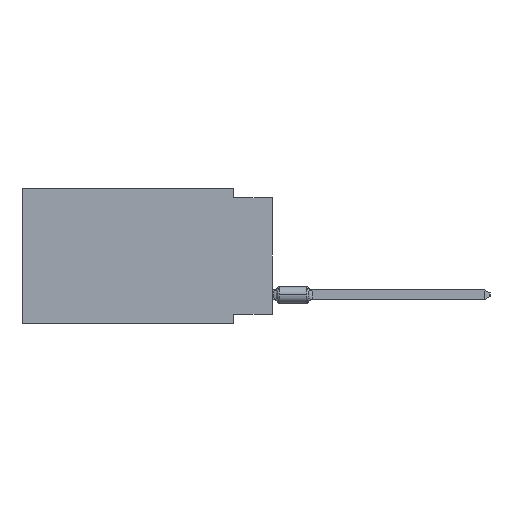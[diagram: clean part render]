
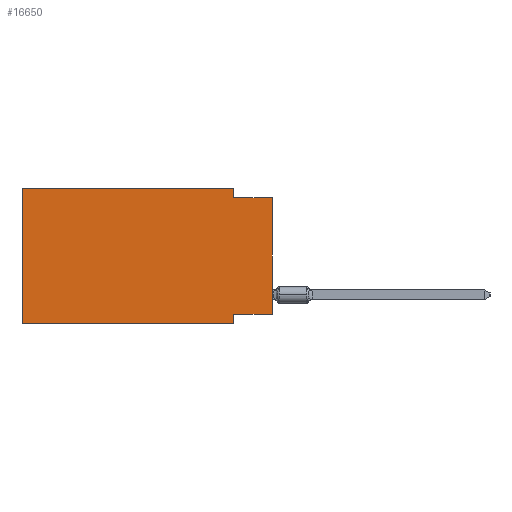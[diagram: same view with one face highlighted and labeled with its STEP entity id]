
A CAD part, left-side view. The second image highlights one B-rep face of the part: STEP entity #16650.
In plain terms, the highlighted planar face has unit normal (-1, 0, 0).
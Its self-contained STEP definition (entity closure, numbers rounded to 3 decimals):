
#592 = FACE_OUTER_BOUND ( 'NONE', #6123, .T. ) ;
#1896 = DIRECTION ( 'NONE',  ( 0., 0., -1. ) ) ;
#2007 = DIRECTION ( 'NONE',  ( 0., -1., 0. ) ) ;
#2099 = VERTEX_POINT ( 'NONE', #8107 ) ;
#2753 = EDGE_CURVE ( 'NONE', #25953, #2099, #21457, .T. ) ;
#3904 = LINE ( 'NONE', #50473, #12168 ) ;
#4431 = ORIENTED_EDGE ( 'NONE', *, *, #30439, .F. ) ;
#4682 = PLANE ( 'NONE',  #30307 ) ;
#4975 = VECTOR ( 'NONE', #37159, 1000. ) ;
#5652 = DIRECTION ( 'NONE',  ( 0., -1., 0. ) ) ;
#5928 = CARTESIAN_POINT ( 'NONE',  ( 0., 16.383, 0. ) ) ;
#6123 = EDGE_LOOP ( 'NONE', ( #35425, #49428, #4431, #21151, #30396, #17695, #19199, #11047 ) ) ;
#6860 = EDGE_CURVE ( 'NONE', #11874, #33828, #3904, .T. ) ;
#8107 = CARTESIAN_POINT ( 'NONE',  ( 0., 2.54, -8.89 ) ) ;
#8528 = DIRECTION ( 'NONE',  ( 0., 0., -1. ) ) ;
#9549 = LINE ( 'NONE', #25925, #24351 ) ;
#10716 = VECTOR ( 'NONE', #47020, 1000. ) ;
#10817 = LINE ( 'NONE', #41771, #4975 ) ;
#10906 = EDGE_CURVE ( 'NONE', #12087, #2099, #9549, .T. ) ;
#11047 = ORIENTED_EDGE ( 'NONE', *, *, #29875, .F. ) ;
#11874 = VERTEX_POINT ( 'NONE', #15835 ) ;
#12087 = VERTEX_POINT ( 'NONE', #13543 ) ;
#12168 = VECTOR ( 'NONE', #46652, 1000. ) ;
#12391 = CARTESIAN_POINT ( 'NONE',  ( 0., 16.383, 0. ) ) ;
#13543 = CARTESIAN_POINT ( 'NONE',  ( 0., 2.54, -8.255 ) ) ;
#15835 = CARTESIAN_POINT ( 'NONE',  ( 0., 2.54, -0.635 ) ) ;
#16650 = ADVANCED_FACE ( 'NONE', ( #592 ), #4682, .F. ) ;
#16654 = LINE ( 'NONE', #28688, #23749 ) ;
#17678 = VECTOR ( 'NONE', #23450, 1000. ) ;
#17695 = ORIENTED_EDGE ( 'NONE', *, *, #2753, .T. ) ;
#18656 = VECTOR ( 'NONE', #18945, 1000. ) ;
#18945 = DIRECTION ( 'NONE',  ( 0., 0., 1. ) ) ;
#19199 = ORIENTED_EDGE ( 'NONE', *, *, #10906, .F. ) ;
#21151 = ORIENTED_EDGE ( 'NONE', *, *, #28235, .F. ) ;
#21457 = LINE ( 'NONE', #37062, #49605 ) ;
#22744 = LINE ( 'NONE', #42179, #10716 ) ;
#23125 = VERTEX_POINT ( 'NONE', #40905 ) ;
#23450 = DIRECTION ( 'NONE',  ( 0., 0., 1. ) ) ;
#23749 = VECTOR ( 'NONE', #5652, 1000. ) ;
#24351 = VECTOR ( 'NONE', #1896, 1000. ) ;
#25925 = CARTESIAN_POINT ( 'NONE',  ( 0., 2.54, -8.89 ) ) ;
#25953 = VERTEX_POINT ( 'NONE', #44857 ) ;
#28235 = EDGE_CURVE ( 'NONE', #41294, #23125, #16654, .T. ) ;
#28688 = CARTESIAN_POINT ( 'NONE',  ( 0., 16.383, 0. ) ) ;
#29875 = EDGE_CURVE ( 'NONE', #43245, #12087, #10817, .T. ) ;
#30213 = LINE ( 'NONE', #45828, #18656 ) ;
#30307 = AXIS2_PLACEMENT_3D ( 'NONE', #12391, #38972, #8528 ) ;
#30396 = ORIENTED_EDGE ( 'NONE', *, *, #50262, .F. ) ;
#30439 = EDGE_CURVE ( 'NONE', #23125, #11874, #22744, .T. ) ;
#33828 = VERTEX_POINT ( 'NONE', #40117 ) ;
#35425 = ORIENTED_EDGE ( 'NONE', *, *, #37527, .T. ) ;
#35718 = CARTESIAN_POINT ( 'NONE',  ( 0., 16.383, 0. ) ) ;
#37062 = CARTESIAN_POINT ( 'NONE',  ( 0., 16.383, -8.89 ) ) ;
#37159 = DIRECTION ( 'NONE',  ( 0., 1., 0. ) ) ;
#37527 = EDGE_CURVE ( 'NONE', #43245, #33828, #30213, .T. ) ;
#38972 = DIRECTION ( 'NONE',  ( 1., 0., 0. ) ) ;
#40117 = CARTESIAN_POINT ( 'NONE',  ( 0., 0., -0.635 ) ) ;
#40905 = CARTESIAN_POINT ( 'NONE',  ( 0., 2.54, 0. ) ) ;
#41294 = VERTEX_POINT ( 'NONE', #5928 ) ;
#41771 = CARTESIAN_POINT ( 'NONE',  ( 0., 0., -8.255 ) ) ;
#42019 = CARTESIAN_POINT ( 'NONE',  ( 0., 0., -8.255 ) ) ;
#42179 = CARTESIAN_POINT ( 'NONE',  ( 0., 2.54, 0. ) ) ;
#43245 = VERTEX_POINT ( 'NONE', #42019 ) ;
#44857 = CARTESIAN_POINT ( 'NONE',  ( 0., 16.383, -8.89 ) ) ;
#45828 = CARTESIAN_POINT ( 'NONE',  ( 0., 0., 0. ) ) ;
#46652 = DIRECTION ( 'NONE',  ( 0., -1., 0. ) ) ;
#47020 = DIRECTION ( 'NONE',  ( 0., 0., -1. ) ) ;
#49428 = ORIENTED_EDGE ( 'NONE', *, *, #6860, .F. ) ;
#49605 = VECTOR ( 'NONE', #2007, 1000. ) ;
#50094 = LINE ( 'NONE', #35718, #17678 ) ;
#50262 = EDGE_CURVE ( 'NONE', #25953, #41294, #50094, .T. ) ;
#50473 = CARTESIAN_POINT ( 'NONE',  ( 0., 0., -0.635 ) ) ;
